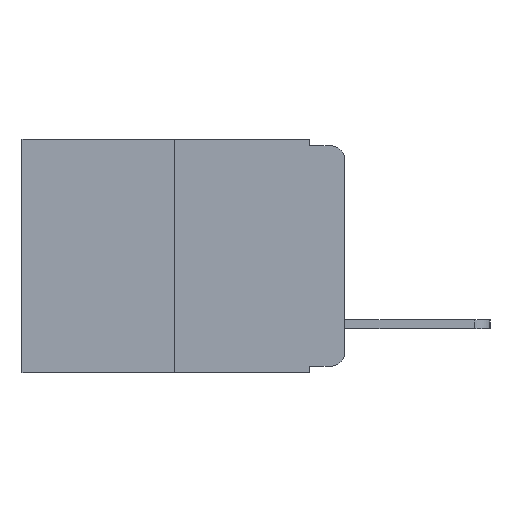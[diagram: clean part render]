
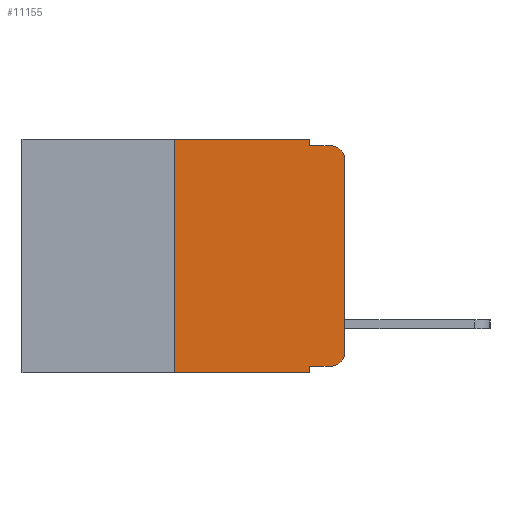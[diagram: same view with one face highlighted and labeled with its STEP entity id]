
A CAD part, left-side view. The second image highlights one B-rep face of the part: STEP entity #11155.
In plain terms, the highlighted planar face has unit normal (-1, 0, 0).
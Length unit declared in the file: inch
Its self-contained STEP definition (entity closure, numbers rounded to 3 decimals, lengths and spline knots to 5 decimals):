
#55 = LINE ( 'NONE', #6211, #7041 ) ;
#104 = CARTESIAN_POINT ( 'NONE',  ( 0., 0., -0.03 ) ) ;
#139 = LINE ( 'NONE', #7231, #9199 ) ;
#299 = VECTOR ( 'NONE', #1914, 39.37008 ) ;
#426 = VERTEX_POINT ( 'NONE', #3972 ) ;
#481 = VERTEX_POINT ( 'NONE', #912 ) ;
#624 = AXIS2_PLACEMENT_3D ( 'NONE', #4416, #10618, #5306 ) ;
#820 = EDGE_CURVE ( 'NONE', #2611, #5188, #4478, .T. ) ;
#876 = ORIENTED_EDGE ( 'NONE', *, *, #6635, .T. ) ;
#912 = CARTESIAN_POINT ( 'NONE',  ( 0., 0.25, -0.343 ) ) ;
#1001 = DIRECTION ( 'NONE',  ( 1., 0., 0. ) ) ;
#1065 = VECTOR ( 'NONE', #3610, 39.37008 ) ;
#1187 = ORIENTED_EDGE ( 'NONE', *, *, #6504, .T. ) ;
#1219 = EDGE_CURVE ( 'NONE', #481, #1745, #5872, .T. ) ;
#1386 = CARTESIAN_POINT ( 'NONE',  ( 0., 0., -0.313 ) ) ;
#1539 = VECTOR ( 'NONE', #8459, 39.37008 ) ;
#1745 = VERTEX_POINT ( 'NONE', #10025 ) ;
#1914 = DIRECTION ( 'NONE',  ( 0., -1., 0. ) ) ;
#1916 = DIRECTION ( 'NONE',  ( 0., -1., 0. ) ) ;
#2031 = VERTEX_POINT ( 'NONE', #10650 ) ;
#2172 = VERTEX_POINT ( 'NONE', #1386 ) ;
#2611 = VERTEX_POINT ( 'NONE', #104 ) ;
#3120 = CARTESIAN_POINT ( 'NONE',  ( 0., 0.051, 0. ) ) ;
#3161 = AXIS2_PLACEMENT_3D ( 'NONE', #3853, #3839, #3306 ) ;
#3255 = VERTEX_POINT ( 'NONE', #5477 ) ;
#3306 = DIRECTION ( 'NONE',  ( 0., 0., -1. ) ) ;
#3610 = DIRECTION ( 'NONE',  ( 0., 0., 1. ) ) ;
#3839 = DIRECTION ( 'NONE',  ( -1., 0., 0. ) ) ;
#3853 = CARTESIAN_POINT ( 'NONE',  ( 0., 0.02, -0.03 ) ) ;
#3898 = VECTOR ( 'NONE', #10688, 39.37008 ) ;
#3972 = CARTESIAN_POINT ( 'NONE',  ( 0., 0.051, -0.01 ) ) ;
#4085 = FACE_OUTER_BOUND ( 'NONE', #9691, .T. ) ;
#4237 = ORIENTED_EDGE ( 'NONE', *, *, #1219, .F. ) ;
#4416 = CARTESIAN_POINT ( 'NONE',  ( 0., 0.02, -0.313 ) ) ;
#4478 = CIRCLE ( 'NONE', #3161, 0.02 ) ;
#4601 = LINE ( 'NONE', #3120, #1539 ) ;
#4733 = CARTESIAN_POINT ( 'NONE',  ( 0., 0.051, -0.01 ) ) ;
#4776 = DIRECTION ( 'NONE',  ( 0., 0., 1. ) ) ;
#4945 = EDGE_CURVE ( 'NONE', #11319, #2031, #55, .T. ) ;
#5095 = ORIENTED_EDGE ( 'NONE', *, *, #7154, .F. ) ;
#5188 = VERTEX_POINT ( 'NONE', #9207 ) ;
#5220 = LINE ( 'NONE', #4733, #299 ) ;
#5264 = VERTEX_POINT ( 'NONE', #9321 ) ;
#5306 = DIRECTION ( 'NONE',  ( 0., 0., -1. ) ) ;
#5477 = CARTESIAN_POINT ( 'NONE',  ( 0., 0.051, 0. ) ) ;
#5605 = VECTOR ( 'NONE', #4776, 39.37008 ) ;
#5607 = VECTOR ( 'NONE', #1916, 39.37008 ) ;
#5760 = EDGE_CURVE ( 'NONE', #426, #5188, #5220, .T. ) ;
#5872 = LINE ( 'NONE', #6543, #5605 ) ;
#5876 = LINE ( 'NONE', #9998, #5607 ) ;
#5887 = ORIENTED_EDGE ( 'NONE', *, *, #7886, .T. ) ;
#6211 = CARTESIAN_POINT ( 'NONE',  ( 0., 0.051, 0. ) ) ;
#6363 = DIRECTION ( 'NONE',  ( 0., -1., 0. ) ) ;
#6482 = CARTESIAN_POINT ( 'NONE',  ( 0., 0.473, 0. ) ) ;
#6504 = EDGE_CURVE ( 'NONE', #5264, #2172, #10193, .T. ) ;
#6543 = CARTESIAN_POINT ( 'NONE',  ( 0., 0.25, 0. ) ) ;
#6635 = EDGE_CURVE ( 'NONE', #481, #2031, #139, .T. ) ;
#6750 = ORIENTED_EDGE ( 'NONE', *, *, #5760, .F. ) ;
#7041 = VECTOR ( 'NONE', #10632, 39.37008 ) ;
#7154 = EDGE_CURVE ( 'NONE', #1745, #3255, #11019, .T. ) ;
#7231 = CARTESIAN_POINT ( 'NONE',  ( 0., 0.473, -0.343 ) ) ;
#7361 = DIRECTION ( 'NONE',  ( 0., 0., -1. ) ) ;
#7886 = EDGE_CURVE ( 'NONE', #11319, #5264, #5876, .T. ) ;
#8459 = DIRECTION ( 'NONE',  ( 0., 0., -1. ) ) ;
#8686 = EDGE_CURVE ( 'NONE', #3255, #426, #4601, .T. ) ;
#9199 = VECTOR ( 'NONE', #6363, 39.37008 ) ;
#9207 = CARTESIAN_POINT ( 'NONE',  ( 0., 0.02, -0.01 ) ) ;
#9321 = CARTESIAN_POINT ( 'NONE',  ( 0., 0.02, -0.333 ) ) ;
#9364 = CARTESIAN_POINT ( 'NONE',  ( 0., 0.051, -0.333 ) ) ;
#9691 = EDGE_LOOP ( 'NONE', ( #11186, #9950, #6750, #10639, #5095, #4237, #876, #11422, #5887, #1187 ) ) ;
#9950 = ORIENTED_EDGE ( 'NONE', *, *, #820, .T. ) ;
#9998 = CARTESIAN_POINT ( 'NONE',  ( 0., 0.051, -0.333 ) ) ;
#10025 = CARTESIAN_POINT ( 'NONE',  ( 0., 0.25, 0. ) ) ;
#10193 = CIRCLE ( 'NONE', #624, 0.02 ) ;
#10356 = EDGE_CURVE ( 'NONE', #2172, #2611, #11488, .T. ) ;
#10478 = AXIS2_PLACEMENT_3D ( 'NONE', #6482, #1001, #7361 ) ;
#10618 = DIRECTION ( 'NONE',  ( -1., 0., 0. ) ) ;
#10632 = DIRECTION ( 'NONE',  ( 0., 0., -1. ) ) ;
#10639 = ORIENTED_EDGE ( 'NONE', *, *, #8686, .F. ) ;
#10650 = CARTESIAN_POINT ( 'NONE',  ( 0., 0.051, -0.343 ) ) ;
#10688 = DIRECTION ( 'NONE',  ( 0., -1., 0. ) ) ;
#10903 = PLANE ( 'NONE',  #10478 ) ;
#11019 = LINE ( 'NONE', #11527, #3898 ) ;
#11155 = ADVANCED_FACE ( 'NONE', ( #4085 ), #10903, .F. ) ;
#11186 = ORIENTED_EDGE ( 'NONE', *, *, #10356, .T. ) ;
#11319 = VERTEX_POINT ( 'NONE', #9364 ) ;
#11422 = ORIENTED_EDGE ( 'NONE', *, *, #4945, .F. ) ;
#11488 = LINE ( 'NONE', #11603, #1065 ) ;
#11527 = CARTESIAN_POINT ( 'NONE',  ( 0., 0.473, 0. ) ) ;
#11603 = CARTESIAN_POINT ( 'NONE',  ( 0., 0., 0. ) ) ;
